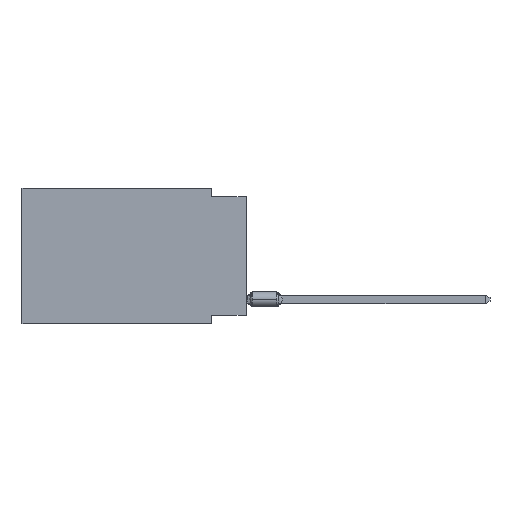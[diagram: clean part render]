
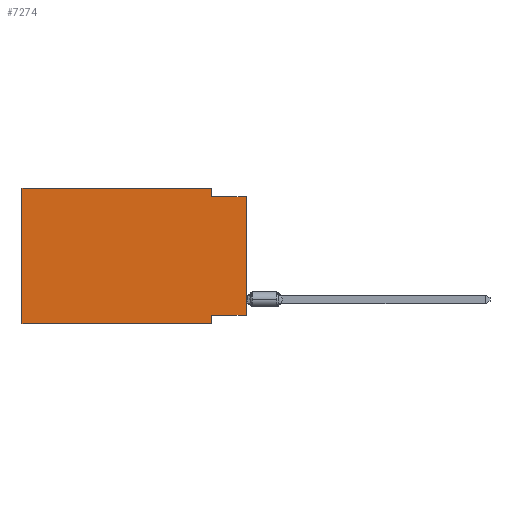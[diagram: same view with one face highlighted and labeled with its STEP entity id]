
A CAD part, left-side view. The second image highlights one B-rep face of the part: STEP entity #7274.
In plain terms, the highlighted planar face has unit normal (-1, 0, 0).
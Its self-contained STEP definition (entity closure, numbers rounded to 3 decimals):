
#101 = VECTOR ( 'NONE', #21250, 1000. ) ;
#457 = DIRECTION ( 'NONE',  ( 0., 0., 1. ) ) ;
#524 = CARTESIAN_POINT ( 'NONE',  ( 0., 16.383, -9.906 ) ) ;
#1192 = CARTESIAN_POINT ( 'NONE',  ( 0., 2.54, -9.906 ) ) ;
#1730 = ORIENTED_EDGE ( 'NONE', *, *, #22813, .F. ) ;
#2601 = VECTOR ( 'NONE', #10689, 1000. ) ;
#2714 = VERTEX_POINT ( 'NONE', #20479 ) ;
#2914 = LINE ( 'NONE', #22741, #7753 ) ;
#2950 = ORIENTED_EDGE ( 'NONE', *, *, #9711, .F. ) ;
#2981 = VECTOR ( 'NONE', #23839, 1000. ) ;
#3554 = LINE ( 'NONE', #15870, #8492 ) ;
#3900 = VECTOR ( 'NONE', #457, 1000. ) ;
#4329 = ORIENTED_EDGE ( 'NONE', *, *, #16269, .F. ) ;
#4763 = LINE ( 'NONE', #20717, #3900 ) ;
#4828 = CARTESIAN_POINT ( 'NONE',  ( 0., 2.54, -0.635 ) ) ;
#5182 = EDGE_CURVE ( 'NONE', #9592, #12781, #3554, .T. ) ;
#6296 = ORIENTED_EDGE ( 'NONE', *, *, #13167, .F. ) ;
#6299 = VERTEX_POINT ( 'NONE', #13342 ) ;
#6443 = CARTESIAN_POINT ( 'NONE',  ( 0., 16.383, 0. ) ) ;
#7274 = ADVANCED_FACE ( 'NONE', ( #20871 ), #16857, .F. ) ;
#7753 = VECTOR ( 'NONE', #20866, 1000. ) ;
#8492 = VECTOR ( 'NONE', #11742, 1000. ) ;
#8797 = LINE ( 'NONE', #16941, #9993 ) ;
#9092 = LINE ( 'NONE', #13081, #101 ) ;
#9363 = VERTEX_POINT ( 'NONE', #524 ) ;
#9592 = VERTEX_POINT ( 'NONE', #25712 ) ;
#9711 = EDGE_CURVE ( 'NONE', #14832, #6299, #15672, .T. ) ;
#9993 = VECTOR ( 'NONE', #12918, 1000. ) ;
#10309 = CARTESIAN_POINT ( 'NONE',  ( 0., 0., -0.635 ) ) ;
#10689 = DIRECTION ( 'NONE',  ( 0., -1., 0. ) ) ;
#11742 = DIRECTION ( 'NONE',  ( 0., 0., -1. ) ) ;
#12103 = VECTOR ( 'NONE', #24339, 1000. ) ;
#12781 = VERTEX_POINT ( 'NONE', #4828 ) ;
#12918 = DIRECTION ( 'NONE',  ( 0., -1., 0. ) ) ;
#13081 = CARTESIAN_POINT ( 'NONE',  ( 0., 16.383, -9.906 ) ) ;
#13167 = EDGE_CURVE ( 'NONE', #6299, #24455, #2914, .T. ) ;
#13342 = CARTESIAN_POINT ( 'NONE',  ( 0., 2.54, -9.271 ) ) ;
#13474 = EDGE_CURVE ( 'NONE', #14832, #2714, #4763, .T. ) ;
#13679 = CARTESIAN_POINT ( 'NONE',  ( 0., 0., -9.271 ) ) ;
#14197 = ORIENTED_EDGE ( 'NONE', *, *, #18447, .T. ) ;
#14832 = VERTEX_POINT ( 'NONE', #13679 ) ;
#14846 = DIRECTION ( 'NONE',  ( 0., 0., -1. ) ) ;
#15672 = LINE ( 'NONE', #16201, #2981 ) ;
#15870 = CARTESIAN_POINT ( 'NONE',  ( 0., 2.54, 0. ) ) ;
#16184 = LINE ( 'NONE', #18467, #12103 ) ;
#16201 = CARTESIAN_POINT ( 'NONE',  ( 0., 0., -9.271 ) ) ;
#16269 = EDGE_CURVE ( 'NONE', #16868, #9592, #8797, .T. ) ;
#16857 = PLANE ( 'NONE',  #17833 ) ;
#16868 = VERTEX_POINT ( 'NONE', #20070 ) ;
#16941 = CARTESIAN_POINT ( 'NONE',  ( 0., 16.383, 0. ) ) ;
#17833 = AXIS2_PLACEMENT_3D ( 'NONE', #6443, #20998, #14846 ) ;
#18245 = ORIENTED_EDGE ( 'NONE', *, *, #5182, .F. ) ;
#18381 = EDGE_CURVE ( 'NONE', #9363, #16868, #16184, .T. ) ;
#18447 = EDGE_CURVE ( 'NONE', #9363, #24455, #9092, .T. ) ;
#18467 = CARTESIAN_POINT ( 'NONE',  ( 0., 16.383, 0. ) ) ;
#20070 = CARTESIAN_POINT ( 'NONE',  ( 0., 16.383, 0. ) ) ;
#20479 = CARTESIAN_POINT ( 'NONE',  ( 0., 0., -0.635 ) ) ;
#20717 = CARTESIAN_POINT ( 'NONE',  ( 0., 0., 0. ) ) ;
#20866 = DIRECTION ( 'NONE',  ( 0., 0., -1. ) ) ;
#20871 = FACE_OUTER_BOUND ( 'NONE', #21148, .T. ) ;
#20998 = DIRECTION ( 'NONE',  ( 1., 0., 0. ) ) ;
#21148 = EDGE_LOOP ( 'NONE', ( #23348, #1730, #18245, #4329, #23564, #14197, #6296, #2950 ) ) ;
#21250 = DIRECTION ( 'NONE',  ( 0., -1., 0. ) ) ;
#22741 = CARTESIAN_POINT ( 'NONE',  ( 0., 2.54, -9.906 ) ) ;
#22813 = EDGE_CURVE ( 'NONE', #12781, #2714, #22854, .T. ) ;
#22854 = LINE ( 'NONE', #10309, #2601 ) ;
#23348 = ORIENTED_EDGE ( 'NONE', *, *, #13474, .T. ) ;
#23564 = ORIENTED_EDGE ( 'NONE', *, *, #18381, .F. ) ;
#23839 = DIRECTION ( 'NONE',  ( 0., 1., 0. ) ) ;
#24339 = DIRECTION ( 'NONE',  ( 0., 0., 1. ) ) ;
#24455 = VERTEX_POINT ( 'NONE', #1192 ) ;
#25712 = CARTESIAN_POINT ( 'NONE',  ( 0., 2.54, 0. ) ) ;
